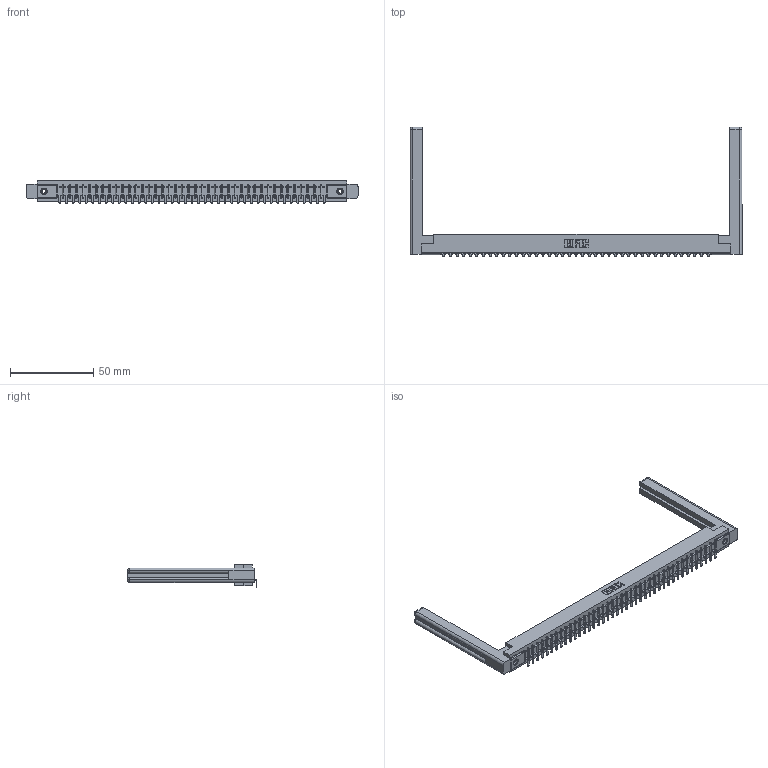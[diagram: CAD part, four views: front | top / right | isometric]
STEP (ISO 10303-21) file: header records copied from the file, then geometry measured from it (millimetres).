
FILE_DESCRIPTION (( 'STEP AP203' ), '1' );
FILE_NAME ('357-041-453-158.STEP', '2020-10-03T08:47:07', ( '' ), ( '' ), 'SwSTEP 2.0', 'SolidWorks 2020', '' );
FILE_SCHEMA (( 'CONFIG_CONTROL_DESIGN' ));
Length unit declared in the file: inch
Products named in the file (5): 307-220-058; 307-290-002_553; 307 Part_.156 Dia Mounting Holes; 345-250-001_345-250-001-102; 357-041-453-158
Assembly tree (46 placements, depth 2):
  357-041-453-158
    307 Part_.156 Dia Mounting Holes
    307-290-002_553  x41
    307-220-058  x2
    345-250-001_345-250-001-102  x2
Bounding box: 199.09 x 77.64 x 13.5 mm (x, y, z)
Volume: 28417.2 mm3; surface area: 31581 mm2
Topology: 46 solids, 46 shells, 3500 faces, 10681 edges, 6994 vertices
Faces by surface type: plane 2081, cylinder 1311, sphere 84, torus 12, cone 12
Entity records: 38759 total; most frequent: CARTESIAN_POINT 6547, ORIENTED_EDGE 6476, DIRECTION 6322, EDGE_CURVE 3238, LINE 2476, VECTOR 2476, VERTEX_POINT 2094, AXIS2_PLACEMENT_3D 1923
